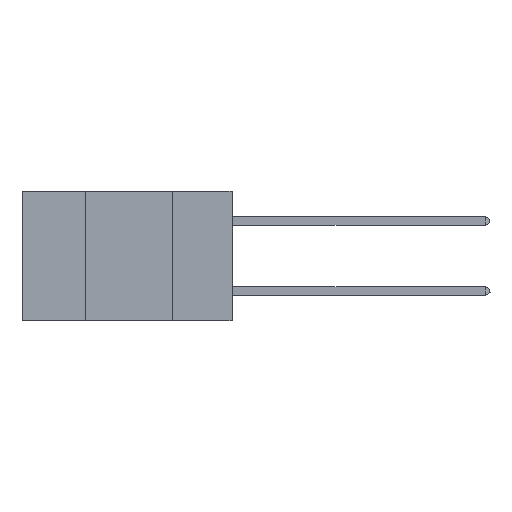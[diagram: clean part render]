
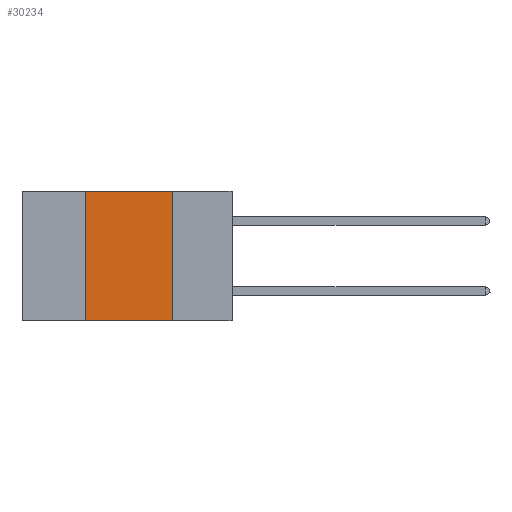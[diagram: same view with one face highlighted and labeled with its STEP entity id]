
A CAD part, left-side view. The second image highlights one B-rep face of the part: STEP entity #30234.
In plain terms, the highlighted planar face has unit normal (-1, 0, 0).
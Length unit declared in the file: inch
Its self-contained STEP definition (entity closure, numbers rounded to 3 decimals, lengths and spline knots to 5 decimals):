
#1058 = CARTESIAN_POINT ( 'NONE',  ( 0., 0.42, 0. ) ) ;
#2545 = DIRECTION ( 'NONE',  ( 0., 0., -1. ) ) ;
#3035 = CARTESIAN_POINT ( 'NONE',  ( 0., 0.42, 0. ) ) ;
#3561 = LINE ( 'NONE', #36987, #11492 ) ;
#4192 = VECTOR ( 'NONE', #2545, 39.37008 ) ;
#4584 = VERTEX_POINT ( 'NONE', #1058 ) ;
#6645 = VECTOR ( 'NONE', #33288, 39.37008 ) ;
#9300 = VERTEX_POINT ( 'NONE', #36180 ) ;
#11492 = VECTOR ( 'NONE', #36406, 39.37008 ) ;
#13122 = EDGE_CURVE ( 'NONE', #4584, #26793, #3561, .T. ) ;
#14396 = VERTEX_POINT ( 'NONE', #31685 ) ;
#15593 = LINE ( 'NONE', #3035, #6645 ) ;
#16152 = CARTESIAN_POINT ( 'NONE',  ( 0., 0.17, 0. ) ) ;
#17912 = DIRECTION ( 'NONE',  ( 1., 0., 0. ) ) ;
#19081 = VECTOR ( 'NONE', #38638, 39.37008 ) ;
#20643 = LINE ( 'NONE', #16152, #4192 ) ;
#24075 = EDGE_LOOP ( 'NONE', ( #38753, #25189, #39004, #34374 ) ) ;
#24446 = CARTESIAN_POINT ( 'NONE',  ( 0., 0.6, 0. ) ) ;
#25189 = ORIENTED_EDGE ( 'NONE', *, *, #13122, .F. ) ;
#26793 = VERTEX_POINT ( 'NONE', #28222 ) ;
#28222 = CARTESIAN_POINT ( 'NONE',  ( 0., 0.17, 0. ) ) ;
#30234 = ADVANCED_FACE ( 'NONE', ( #42237 ), #34567, .F. ) ;
#31685 = CARTESIAN_POINT ( 'NONE',  ( 0., 0.42, -0.37 ) ) ;
#31838 = LINE ( 'NONE', #41312, #19081 ) ;
#33288 = DIRECTION ( 'NONE',  ( 0., 0., 1. ) ) ;
#34374 = ORIENTED_EDGE ( 'NONE', *, *, #42204, .T. ) ;
#34567 = PLANE ( 'NONE',  #37390 ) ;
#35331 = EDGE_CURVE ( 'NONE', #26793, #9300, #20643, .T. ) ;
#36180 = CARTESIAN_POINT ( 'NONE',  ( 0., 0.17, -0.37 ) ) ;
#36406 = DIRECTION ( 'NONE',  ( 0., -1., 0. ) ) ;
#36987 = CARTESIAN_POINT ( 'NONE',  ( 0., 0.6, 0. ) ) ;
#37390 = AXIS2_PLACEMENT_3D ( 'NONE', #24446, #17912, #37980 ) ;
#37980 = DIRECTION ( 'NONE',  ( 0., 0., -1. ) ) ;
#38638 = DIRECTION ( 'NONE',  ( 0., -1., 0. ) ) ;
#38753 = ORIENTED_EDGE ( 'NONE', *, *, #35331, .F. ) ;
#39004 = ORIENTED_EDGE ( 'NONE', *, *, #42641, .F. ) ;
#41312 = CARTESIAN_POINT ( 'NONE',  ( 0., 0.6, -0.37 ) ) ;
#42204 = EDGE_CURVE ( 'NONE', #14396, #9300, #31838, .T. ) ;
#42237 = FACE_OUTER_BOUND ( 'NONE', #24075, .T. ) ;
#42641 = EDGE_CURVE ( 'NONE', #14396, #4584, #15593, .T. ) ;
